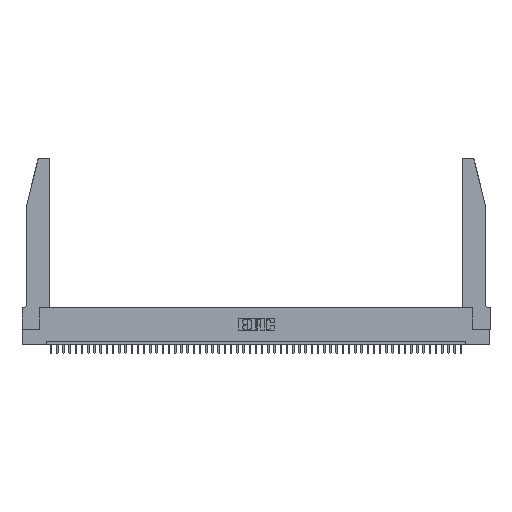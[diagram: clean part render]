
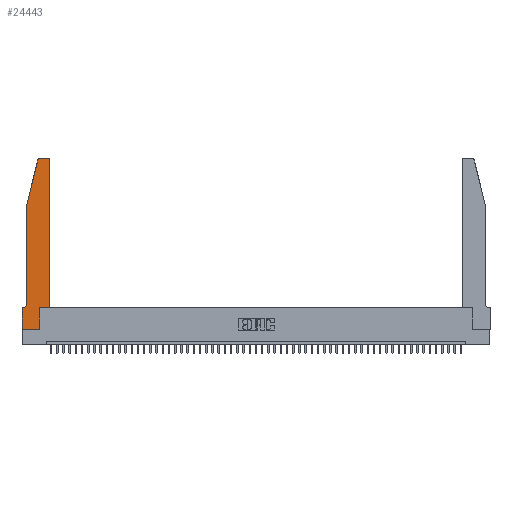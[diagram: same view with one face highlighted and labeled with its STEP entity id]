
A CAD part, top view. The second image highlights one B-rep face of the part: STEP entity #24443.
In plain terms, the highlighted planar face has unit normal (0, 0, 1).
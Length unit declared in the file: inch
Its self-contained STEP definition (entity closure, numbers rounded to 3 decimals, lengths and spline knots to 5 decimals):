
#541 = VERTEX_POINT ( 'NONE', #23976 ) ;
#996 = EDGE_CURVE ( 'NONE', #10154, #39072, #2552, .T. ) ;
#1205 = DIRECTION ( 'NONE',  ( 1., 0., 0. ) ) ;
#2470 = DIRECTION ( 'NONE',  ( 0., 1., 0. ) ) ;
#2552 = LINE ( 'NONE', #31551, #12530 ) ;
#2643 = AXIS2_PLACEMENT_3D ( 'NONE', #48959, #29236, #25081 ) ;
#3000 = LINE ( 'NONE', #51471, #25584 ) ;
#3590 = DIRECTION ( 'NONE',  ( 0., 0., 1. ) ) ;
#5704 = CARTESIAN_POINT ( 'NONE',  ( 0.4505, 0.35, 0.37 ) ) ;
#6095 = CARTESIAN_POINT ( 'NONE',  ( 0.2865, 0.35, 0.37 ) ) ;
#6393 = VERTEX_POINT ( 'NONE', #27807 ) ;
#7137 = DIRECTION ( 'NONE',  ( 0., 1., 0. ) ) ;
#7206 = VERTEX_POINT ( 'NONE', #28905 ) ;
#7301 = VECTOR ( 'NONE', #7137, 39.37008 ) ;
#8129 = ORIENTED_EDGE ( 'NONE', *, *, #50636, .T. ) ;
#8285 = EDGE_CURVE ( 'NONE', #16499, #6393, #3000, .T. ) ;
#8312 = CARTESIAN_POINT ( 'NONE',  ( 0.4505, 2.72, 0.37 ) ) ;
#8553 = ORIENTED_EDGE ( 'NONE', *, *, #40193, .T. ) ;
#9429 = CARTESIAN_POINT ( 'NONE',  ( 0.25487, 2.72718, 0.37 ) ) ;
#9493 = VERTEX_POINT ( 'NONE', #5704 ) ;
#9948 = CARTESIAN_POINT ( 'NONE',  ( 0.0055, 0.35, 0.37 ) ) ;
#10154 = VERTEX_POINT ( 'NONE', #45566 ) ;
#12530 = VECTOR ( 'NONE', #26896, 39.37008 ) ;
#13131 = ORIENTED_EDGE ( 'NONE', *, *, #29594, .T. ) ;
#13332 = PLANE ( 'NONE',  #44322 ) ;
#15308 = VERTEX_POINT ( 'NONE', #42796 ) ;
#15378 = CIRCLE ( 'NONE', #2643, 0.07 ) ;
#16499 = VERTEX_POINT ( 'NONE', #28125 ) ;
#16980 = DIRECTION ( 'NONE',  ( -1., 0., 0. ) ) ;
#17020 = CARTESIAN_POINT ( 'NONE',  ( 0.0755, 2., 0.37 ) ) ;
#17293 = ORIENTED_EDGE ( 'NONE', *, *, #18524, .T. ) ;
#17531 = VERTEX_POINT ( 'NONE', #23548 ) ;
#18003 = LINE ( 'NONE', #6095, #7301 ) ;
#18410 = ORIENTED_EDGE ( 'NONE', *, *, #996, .T. ) ;
#18524 = EDGE_CURVE ( 'NONE', #39072, #15308, #29234, .T. ) ;
#20435 = CIRCLE ( 'NONE', #42832, 0.03 ) ;
#21205 = EDGE_CURVE ( 'NONE', #17531, #9493, #24007, .T. ) ;
#21252 = CARTESIAN_POINT ( 'NONE',  ( 0., 0.35, 0.37 ) ) ;
#23548 = CARTESIAN_POINT ( 'NONE',  ( 0.2865, 0.35, 0.37 ) ) ;
#23601 = DIRECTION ( 'NONE',  ( 1., 0., 0. ) ) ;
#23676 = CARTESIAN_POINT ( 'NONE',  ( 0.4205, 2.72, 0.37 ) ) ;
#23976 = CARTESIAN_POINT ( 'NONE',  ( 0.0755, 2., 0.37 ) ) ;
#24007 = LINE ( 'NONE', #36243, #43921 ) ;
#24124 = ORIENTED_EDGE ( 'NONE', *, *, #50997, .T. ) ;
#24443 = ADVANCED_FACE ( 'NONE', ( #34964 ), #13332, .T. ) ;
#25081 = DIRECTION ( 'NONE',  ( -1., 0., 0. ) ) ;
#25268 = DIRECTION ( 'NONE',  ( 0., 0., 1. ) ) ;
#25584 = VECTOR ( 'NONE', #35600, 39.37008 ) ;
#26896 = DIRECTION ( 'NONE',  ( 0., -1., 0. ) ) ;
#27741 = CIRCLE ( 'NONE', #34566, 0.03 ) ;
#27807 = CARTESIAN_POINT ( 'NONE',  ( 0.284, 2.75, 0.37 ) ) ;
#28018 = VECTOR ( 'NONE', #23601, 39.37008 ) ;
#28125 = CARTESIAN_POINT ( 'NONE',  ( 0.4205, 2.75, 0.37 ) ) ;
#28347 = VECTOR ( 'NONE', #2470, 39.37008 ) ;
#28905 = CARTESIAN_POINT ( 'NONE',  ( 0.0755, 0.42, 0.37 ) ) ;
#29234 = LINE ( 'NONE', #47453, #28018 ) ;
#29236 = DIRECTION ( 'NONE',  ( 0., 0., -1. ) ) ;
#29277 = CARTESIAN_POINT ( 'NONE',  ( 0.0755, 2., 0.37 ) ) ;
#29548 = DIRECTION ( 'NONE',  ( 1., 0., 0. ) ) ;
#29594 = EDGE_CURVE ( 'NONE', #541, #7206, #43783, .T. ) ;
#30598 = VERTEX_POINT ( 'NONE', #9429 ) ;
#30798 = VERTEX_POINT ( 'NONE', #8312 ) ;
#31551 = CARTESIAN_POINT ( 'NONE',  ( 0., 0., 0.37 ) ) ;
#32081 = ORIENTED_EDGE ( 'NONE', *, *, #21205, .T. ) ;
#32589 = ORIENTED_EDGE ( 'NONE', *, *, #42045, .T. ) ;
#32746 = ORIENTED_EDGE ( 'NONE', *, *, #35491, .T. ) ;
#33138 = VECTOR ( 'NONE', #33837, 39.37008 ) ;
#33837 = DIRECTION ( 'NONE',  ( 0., -1., 0. ) ) ;
#34566 = AXIS2_PLACEMENT_3D ( 'NONE', #49444, #45426, #29548 ) ;
#34679 = CARTESIAN_POINT ( 'NONE',  ( 0.0755, 0.35, 0.37 ) ) ;
#34964 = FACE_OUTER_BOUND ( 'NONE', #38302, .T. ) ;
#35491 = EDGE_CURVE ( 'NONE', #30798, #16499, #20435, .T. ) ;
#35600 = DIRECTION ( 'NONE',  ( -1., 0., 0. ) ) ;
#35661 = DIRECTION ( 'NONE',  ( 1., 0., 0. ) ) ;
#35957 = VECTOR ( 'NONE', #36284, 39.37008 ) ;
#36243 = CARTESIAN_POINT ( 'NONE',  ( 0.4505, 0.35, 0.37 ) ) ;
#36284 = DIRECTION ( 'NONE',  ( -0.239, -0.971, 0. ) ) ;
#38302 = EDGE_LOOP ( 'NONE', ( #42199, #24124, #32589, #13131, #42958, #43143, #18410, #17293, #8553, #32081, #8129, #32746 ) ) ;
#39072 = VERTEX_POINT ( 'NONE', #41964 ) ;
#40138 = VERTEX_POINT ( 'NONE', #9948 ) ;
#40193 = EDGE_CURVE ( 'NONE', #15308, #17531, #18003, .T. ) ;
#41563 = LINE ( 'NONE', #34679, #47835 ) ;
#41746 = EDGE_CURVE ( 'NONE', #40138, #10154, #41563, .T. ) ;
#41964 = CARTESIAN_POINT ( 'NONE',  ( 0., 0., 0.37 ) ) ;
#42045 = EDGE_CURVE ( 'NONE', #30598, #541, #46586, .T. ) ;
#42199 = ORIENTED_EDGE ( 'NONE', *, *, #8285, .T. ) ;
#42796 = CARTESIAN_POINT ( 'NONE',  ( 0.2865, 0., 0.37 ) ) ;
#42832 = AXIS2_PLACEMENT_3D ( 'NONE', #23676, #3590, #35661 ) ;
#42958 = ORIENTED_EDGE ( 'NONE', *, *, #49339, .T. ) ;
#43143 = ORIENTED_EDGE ( 'NONE', *, *, #41746, .T. ) ;
#43783 = LINE ( 'NONE', #29277, #33138 ) ;
#43921 = VECTOR ( 'NONE', #44751, 39.37008 ) ;
#44322 = AXIS2_PLACEMENT_3D ( 'NONE', #21252, #25268, #1205 ) ;
#44751 = DIRECTION ( 'NONE',  ( 1., 0., 0. ) ) ;
#45426 = DIRECTION ( 'NONE',  ( 0., 0., 1. ) ) ;
#45566 = CARTESIAN_POINT ( 'NONE',  ( 0., 0.35, 0.37 ) ) ;
#46390 = CARTESIAN_POINT ( 'NONE',  ( 0.4505, 0.35, 0.37 ) ) ;
#46586 = LINE ( 'NONE', #17020, #35957 ) ;
#47107 = LINE ( 'NONE', #46390, #28347 ) ;
#47453 = CARTESIAN_POINT ( 'NONE',  ( 0., 0., 0.37 ) ) ;
#47835 = VECTOR ( 'NONE', #16980, 39.37008 ) ;
#48959 = CARTESIAN_POINT ( 'NONE',  ( 0.0055, 0.42, 0.37 ) ) ;
#49339 = EDGE_CURVE ( 'NONE', #7206, #40138, #15378, .T. ) ;
#49444 = CARTESIAN_POINT ( 'NONE',  ( 0.284, 2.72, 0.37 ) ) ;
#50636 = EDGE_CURVE ( 'NONE', #9493, #30798, #47107, .T. ) ;
#50997 = EDGE_CURVE ( 'NONE', #6393, #30598, #27741, .T. ) ;
#51471 = CARTESIAN_POINT ( 'NONE',  ( 0.2605, 2.75, 0.37 ) ) ;
